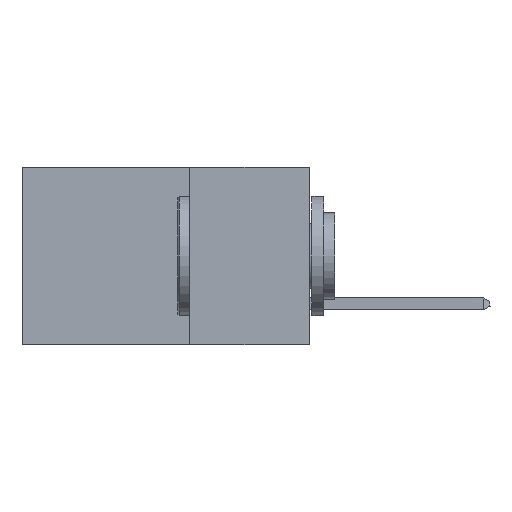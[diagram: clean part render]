
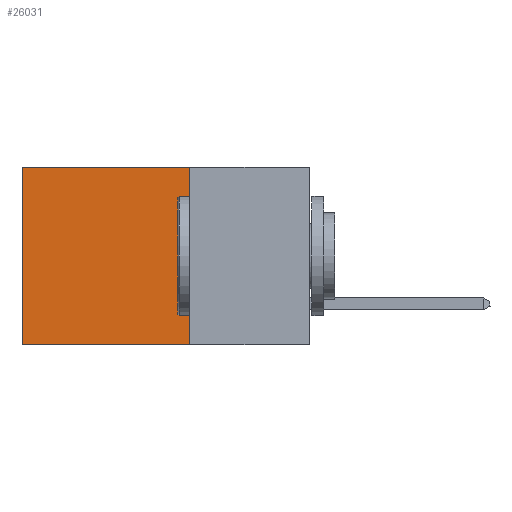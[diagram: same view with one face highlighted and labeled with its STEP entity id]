
A CAD part, left-side view. The second image highlights one B-rep face of the part: STEP entity #26031.
In plain terms, the highlighted planar face has unit normal (-1, 0, 0).
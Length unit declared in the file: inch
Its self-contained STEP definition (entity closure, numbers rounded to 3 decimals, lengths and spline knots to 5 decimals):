
#1757 = CARTESIAN_POINT ( 'NONE',  ( 0.2875, 0.6, -0.37 ) ) ;
#1928 = DIRECTION ( 'NONE',  ( 0., 0., -1. ) ) ;
#2193 = EDGE_CURVE ( 'NONE', #2914, #18800, #5655, .T. ) ;
#2472 = CARTESIAN_POINT ( 'NONE',  ( 0.2875, 0.25, -0.37 ) ) ;
#2914 = VERTEX_POINT ( 'NONE', #23840 ) ;
#4033 = DIRECTION ( 'NONE',  ( 0., 1., 0. ) ) ;
#5655 = LINE ( 'NONE', #11534, #33398 ) ;
#5943 = LINE ( 'NONE', #39072, #13698 ) ;
#6054 = LINE ( 'NONE', #27550, #24557 ) ;
#7511 = ORIENTED_EDGE ( 'NONE', *, *, #36175, .F. ) ;
#8485 = ORIENTED_EDGE ( 'NONE', *, *, #12859, .T. ) ;
#10339 = AXIS2_PLACEMENT_3D ( 'NONE', #11628, #26845, #17874 ) ;
#10817 = DIRECTION ( 'NONE',  ( 0., 0., -1. ) ) ;
#10877 = FACE_OUTER_BOUND ( 'NONE', #16689, .T. ) ;
#11021 = VERTEX_POINT ( 'NONE', #1757 ) ;
#11534 = CARTESIAN_POINT ( 'NONE',  ( 0.2875, 0.25, 0. ) ) ;
#11628 = CARTESIAN_POINT ( 'NONE',  ( 0.2875, 0.25, 0. ) ) ;
#12859 = EDGE_CURVE ( 'NONE', #2914, #38526, #6054, .T. ) ;
#13698 = VECTOR ( 'NONE', #10817, 39.37008 ) ;
#16689 = EDGE_LOOP ( 'NONE', ( #27073, #7511, #25454, #8485 ) ) ;
#17874 = DIRECTION ( 'NONE',  ( 0., 0., -1. ) ) ;
#18800 = VERTEX_POINT ( 'NONE', #2472 ) ;
#19576 = CARTESIAN_POINT ( 'NONE',  ( 0.2875, 0.25, -0.37 ) ) ;
#21384 = EDGE_CURVE ( 'NONE', #38526, #11021, #5943, .T. ) ;
#23840 = CARTESIAN_POINT ( 'NONE',  ( 0.2875, 0.25, 0. ) ) ;
#24557 = VECTOR ( 'NONE', #39753, 39.37008 ) ;
#25261 = CARTESIAN_POINT ( 'NONE',  ( 0.2875, 0.6, 0. ) ) ;
#25454 = ORIENTED_EDGE ( 'NONE', *, *, #2193, .F. ) ;
#26031 = ADVANCED_FACE ( 'NONE', ( #10877 ), #30363, .F. ) ;
#26845 = DIRECTION ( 'NONE',  ( 1., 0., 0. ) ) ;
#27073 = ORIENTED_EDGE ( 'NONE', *, *, #21384, .T. ) ;
#27550 = CARTESIAN_POINT ( 'NONE',  ( 0.2875, 0.25, 0. ) ) ;
#30363 = PLANE ( 'NONE',  #10339 ) ;
#33398 = VECTOR ( 'NONE', #1928, 39.37008 ) ;
#36175 = EDGE_CURVE ( 'NONE', #18800, #11021, #36810, .T. ) ;
#36810 = LINE ( 'NONE', #19576, #39731 ) ;
#38526 = VERTEX_POINT ( 'NONE', #25261 ) ;
#39072 = CARTESIAN_POINT ( 'NONE',  ( 0.2875, 0.6, 0. ) ) ;
#39731 = VECTOR ( 'NONE', #4033, 39.37008 ) ;
#39753 = DIRECTION ( 'NONE',  ( 0., 1., 0. ) ) ;
